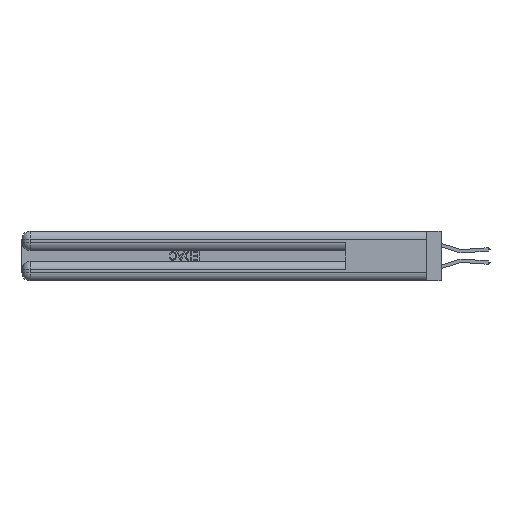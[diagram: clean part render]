
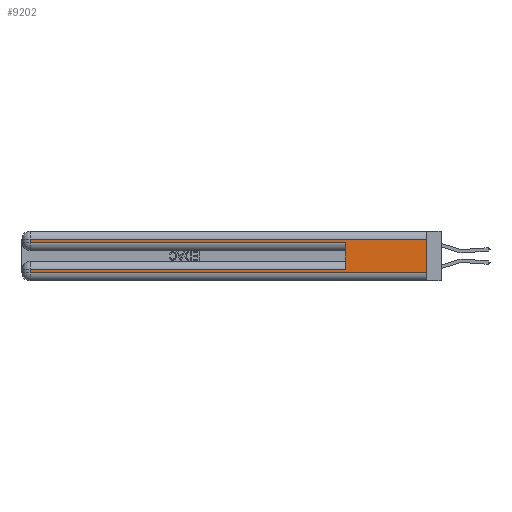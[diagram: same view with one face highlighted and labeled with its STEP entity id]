
A CAD part, left-side view. The second image highlights one B-rep face of the part: STEP entity #9202.
In plain terms, the highlighted planar face has unit normal (-1, 0, 0).
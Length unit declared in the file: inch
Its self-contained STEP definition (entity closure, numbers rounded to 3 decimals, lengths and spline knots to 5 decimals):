
#26 = DIRECTION ( 'NONE',  ( 0., 0., -1. ) ) ;
#1088 = DIRECTION ( 'NONE',  ( 0., 0., 1. ) ) ;
#1208 = CARTESIAN_POINT ( 'NONE',  ( 0., 0., 0.37 ) ) ;
#1594 = VECTOR ( 'NONE', #8582, 39.37008 ) ;
#4266 = LINE ( 'NONE', #15918, #12509 ) ;
#4637 = ORIENTED_EDGE ( 'NONE', *, *, #33066, .F. ) ;
#4852 = DIRECTION ( 'NONE',  ( 0., 0., -1. ) ) ;
#5750 = CARTESIAN_POINT ( 'NONE',  ( 0., 0., 0.06 ) ) ;
#5859 = CARTESIAN_POINT ( 'NONE',  ( 0., 0., 0.06 ) ) ;
#6785 = CARTESIAN_POINT ( 'NONE',  ( 0., 2.94, 0.37 ) ) ;
#7494 = CARTESIAN_POINT ( 'NONE',  ( 0., 2.94, 0.285 ) ) ;
#7998 = CARTESIAN_POINT ( 'NONE',  ( 0., 0.6, 0.145 ) ) ;
#8270 = DIRECTION ( 'NONE',  ( 1., 0., 0. ) ) ;
#8384 = LINE ( 'NONE', #7998, #44680 ) ;
#8480 = ORIENTED_EDGE ( 'NONE', *, *, #40852, .T. ) ;
#8582 = DIRECTION ( 'NONE',  ( 0., 1., 0. ) ) ;
#9024 = VECTOR ( 'NONE', #9300, 39.37008 ) ;
#9125 = EDGE_LOOP ( 'NONE', ( #4637, #24536, #9477, #30365, #15531, #40070, #8480, #42494 ) ) ;
#9179 = VERTEX_POINT ( 'NONE', #29222 ) ;
#9202 = ADVANCED_FACE ( 'NONE', ( #22209 ), #29389, .F. ) ;
#9300 = DIRECTION ( 'NONE',  ( 0., -1., 0. ) ) ;
#9477 = ORIENTED_EDGE ( 'NONE', *, *, #10172, .T. ) ;
#10020 = VERTEX_POINT ( 'NONE', #5859 ) ;
#10172 = EDGE_CURVE ( 'NONE', #9179, #32966, #44594, .T. ) ;
#11088 = AXIS2_PLACEMENT_3D ( 'NONE', #1208, #8270, #32909 ) ;
#11241 = EDGE_CURVE ( 'NONE', #26726, #9179, #29701, .T. ) ;
#12278 = LINE ( 'NONE', #21750, #39288 ) ;
#12509 = VECTOR ( 'NONE', #44073, 39.37008 ) ;
#13186 = EDGE_CURVE ( 'NONE', #32966, #26066, #12278, .T. ) ;
#15531 = ORIENTED_EDGE ( 'NONE', *, *, #25775, .F. ) ;
#15918 = CARTESIAN_POINT ( 'NONE',  ( 0., 2.94, 0.37 ) ) ;
#17496 = VERTEX_POINT ( 'NONE', #43306 ) ;
#19069 = CARTESIAN_POINT ( 'NONE',  ( 0., 0., 0.31 ) ) ;
#21750 = CARTESIAN_POINT ( 'NONE',  ( 0., 0., 0.285 ) ) ;
#21850 = CARTESIAN_POINT ( 'NONE',  ( 0., 2.94, 0.085 ) ) ;
#22209 = FACE_OUTER_BOUND ( 'NONE', #9125, .T. ) ;
#24536 = ORIENTED_EDGE ( 'NONE', *, *, #11241, .T. ) ;
#25775 = EDGE_CURVE ( 'NONE', #31711, #26066, #8384, .T. ) ;
#26066 = VERTEX_POINT ( 'NONE', #30920 ) ;
#26726 = VERTEX_POINT ( 'NONE', #39906 ) ;
#28144 = VECTOR ( 'NONE', #26, 39.37008 ) ;
#28181 = VECTOR ( 'NONE', #4852, 39.37008 ) ;
#28820 = DIRECTION ( 'NONE',  ( 0., -1., 0. ) ) ;
#28926 = CARTESIAN_POINT ( 'NONE',  ( 0., 0., 0.085 ) ) ;
#29209 = CARTESIAN_POINT ( 'NONE',  ( 0., 0., 0.37 ) ) ;
#29222 = CARTESIAN_POINT ( 'NONE',  ( 0., 2.94, 0.31 ) ) ;
#29389 = PLANE ( 'NONE',  #11088 ) ;
#29701 = LINE ( 'NONE', #19069, #1594 ) ;
#30365 = ORIENTED_EDGE ( 'NONE', *, *, #13186, .T. ) ;
#30920 = CARTESIAN_POINT ( 'NONE',  ( 0., 0.6, 0.285 ) ) ;
#31711 = VERTEX_POINT ( 'NONE', #33366 ) ;
#31825 = EDGE_CURVE ( 'NONE', #17496, #10020, #45310, .T. ) ;
#32909 = DIRECTION ( 'NONE',  ( 0., 0., -1. ) ) ;
#32966 = VERTEX_POINT ( 'NONE', #7494 ) ;
#33066 = EDGE_CURVE ( 'NONE', #26726, #10020, #37544, .T. ) ;
#33366 = CARTESIAN_POINT ( 'NONE',  ( 0., 0.6, 0.085 ) ) ;
#34938 = EDGE_CURVE ( 'NONE', #31711, #38618, #45525, .T. ) ;
#37544 = LINE ( 'NONE', #29209, #28181 ) ;
#38618 = VERTEX_POINT ( 'NONE', #21850 ) ;
#39288 = VECTOR ( 'NONE', #28820, 39.37008 ) ;
#39906 = CARTESIAN_POINT ( 'NONE',  ( 0., 0., 0.31 ) ) ;
#40070 = ORIENTED_EDGE ( 'NONE', *, *, #34938, .T. ) ;
#40852 = EDGE_CURVE ( 'NONE', #38618, #17496, #4266, .T. ) ;
#42494 = ORIENTED_EDGE ( 'NONE', *, *, #31825, .T. ) ;
#43058 = DIRECTION ( 'NONE',  ( 0., 1., 0. ) ) ;
#43306 = CARTESIAN_POINT ( 'NONE',  ( 0., 2.94, 0.06 ) ) ;
#44073 = DIRECTION ( 'NONE',  ( 0., 0., -1. ) ) ;
#44455 = VECTOR ( 'NONE', #43058, 39.37008 ) ;
#44594 = LINE ( 'NONE', #6785, #28144 ) ;
#44680 = VECTOR ( 'NONE', #1088, 39.37008 ) ;
#45310 = LINE ( 'NONE', #5750, #9024 ) ;
#45525 = LINE ( 'NONE', #28926, #44455 ) ;
